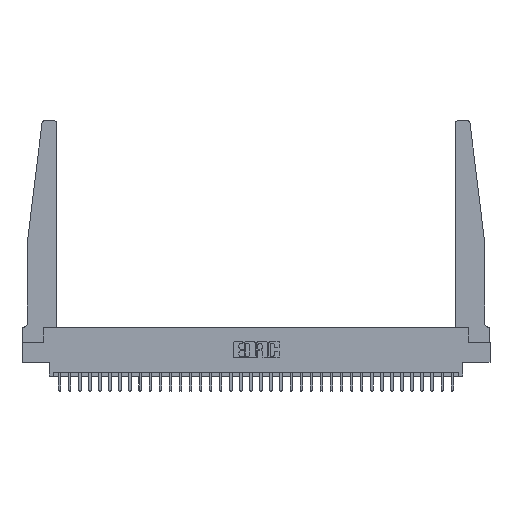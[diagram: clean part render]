
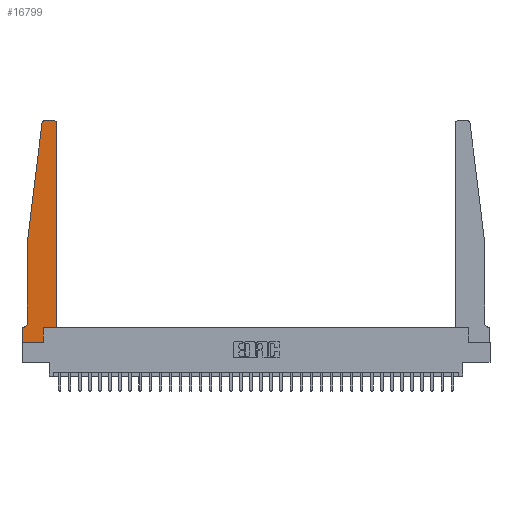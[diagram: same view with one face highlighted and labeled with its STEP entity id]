
A CAD part, top view. The second image highlights one B-rep face of the part: STEP entity #16799.
In plain terms, the highlighted planar face has unit normal (0, 0, 1).
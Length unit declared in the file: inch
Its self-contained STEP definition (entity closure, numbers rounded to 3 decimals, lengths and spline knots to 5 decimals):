
#183 = DIRECTION ( 'NONE',  ( 0., -1., 0. ) ) ;
#861 = EDGE_CURVE ( 'NONE', #28342, #23080, #4961, .T. ) ;
#1262 = VECTOR ( 'NONE', #183, 39.37008 ) ;
#2388 = VERTEX_POINT ( 'NONE', #28001 ) ;
#2410 = DIRECTION ( 'NONE',  ( -1., 0., 0. ) ) ;
#2727 = CARTESIAN_POINT ( 'NONE',  ( 0.2605, 0., 0.37 ) ) ;
#2827 = VECTOR ( 'NONE', #9152, 39.37008 ) ;
#3129 = VERTEX_POINT ( 'NONE', #16796 ) ;
#3364 = EDGE_CURVE ( 'NONE', #8021, #3392, #20960, .T. ) ;
#3392 = VERTEX_POINT ( 'NONE', #20138 ) ;
#3510 = DIRECTION ( 'NONE',  ( -0.122, -0.992, 0. ) ) ;
#4955 = CARTESIAN_POINT ( 'NONE',  ( 0.25, 2.75, 0.37 ) ) ;
#4961 = LINE ( 'NONE', #15987, #18856 ) ;
#5019 = VERTEX_POINT ( 'NONE', #28207 ) ;
#5576 = EDGE_CURVE ( 'NONE', #5019, #2388, #22667, .T. ) ;
#5673 = EDGE_CURVE ( 'NONE', #22853, #3129, #7489, .T. ) ;
#5853 = CARTESIAN_POINT ( 'NONE',  ( 0.065, 1.25, 0.37 ) ) ;
#6017 = ORIENTED_EDGE ( 'NONE', *, *, #10402, .T. ) ;
#6087 = CARTESIAN_POINT ( 'NONE',  ( 0.395, 2.72, 0.37 ) ) ;
#7252 = ORIENTED_EDGE ( 'NONE', *, *, #5576, .T. ) ;
#7489 = LINE ( 'NONE', #21246, #20468 ) ;
#7594 = ORIENTED_EDGE ( 'NONE', *, *, #5673, .T. ) ;
#7790 = VECTOR ( 'NONE', #22887, 39.37008 ) ;
#8021 = VERTEX_POINT ( 'NONE', #10655 ) ;
#8099 = CARTESIAN_POINT ( 'NONE',  ( 0.27653, 2.72, 0.37 ) ) ;
#8531 = LINE ( 'NONE', #4955, #20725 ) ;
#8535 = CARTESIAN_POINT ( 'NONE',  ( 0.015, 0.2375, 0.37 ) ) ;
#8607 = DIRECTION ( 'NONE',  ( 1., 0., 0. ) ) ;
#8812 = PLANE ( 'NONE',  #18573 ) ;
#9152 = DIRECTION ( 'NONE',  ( -1., 0., 0. ) ) ;
#9155 = DIRECTION ( 'NONE',  ( 1., 0., 0. ) ) ;
#9532 = LINE ( 'NONE', #18881, #2827 ) ;
#10249 = CARTESIAN_POINT ( 'NONE',  ( 0., 0., 0.37 ) ) ;
#10363 = LINE ( 'NONE', #22109, #22428 ) ;
#10402 = EDGE_CURVE ( 'NONE', #22274, #21176, #17820, .T. ) ;
#10571 = VERTEX_POINT ( 'NONE', #30438 ) ;
#10602 = DIRECTION ( 'NONE',  ( 1., 0., 0. ) ) ;
#10638 = ORIENTED_EDGE ( 'NONE', *, *, #13900, .T. ) ;
#10655 = CARTESIAN_POINT ( 'NONE',  ( 0., 0.1875, 0.37 ) ) ;
#11037 = DIRECTION ( 'NONE',  ( -1., 0., 0. ) ) ;
#11327 = DIRECTION ( 'NONE',  ( 1., 0., 0. ) ) ;
#12729 = ORIENTED_EDGE ( 'NONE', *, *, #31238, .T. ) ;
#13421 = CARTESIAN_POINT ( 'NONE',  ( 0.425, 0.18, 0.37 ) ) ;
#13825 = CARTESIAN_POINT ( 'NONE',  ( 0.24675, 2.72367, 0.37 ) ) ;
#13900 = EDGE_CURVE ( 'NONE', #24405, #22853, #19134, .T. ) ;
#14165 = CARTESIAN_POINT ( 'NONE',  ( 0.2605, 0.18, 0.37 ) ) ;
#14220 = CARTESIAN_POINT ( 'NONE',  ( 0.065, 0.2375, 0.37 ) ) ;
#15987 = CARTESIAN_POINT ( 'NONE',  ( 0.065, 1.25, 0.37 ) ) ;
#16172 = CARTESIAN_POINT ( 'NONE',  ( 0., 0.1875, 0.37 ) ) ;
#16620 = DIRECTION ( 'NONE',  ( 0., 1., 0. ) ) ;
#16796 = CARTESIAN_POINT ( 'NONE',  ( 0.425, 0.18, 0.37 ) ) ;
#16799 = ADVANCED_FACE ( 'NONE', ( #20172 ), #8812, .T. ) ;
#17820 = CIRCLE ( 'NONE', #19239, 0.05 ) ;
#17997 = EDGE_CURVE ( 'NONE', #3129, #5019, #25944, .T. ) ;
#18573 = AXIS2_PLACEMENT_3D ( 'NONE', #16172, #25641, #11327 ) ;
#18640 = CARTESIAN_POINT ( 'NONE',  ( 0.2605, 0.18, 0.37 ) ) ;
#18856 = VECTOR ( 'NONE', #3510, 39.37008 ) ;
#18881 = CARTESIAN_POINT ( 'NONE',  ( 0.065, 0.1875, 0.37 ) ) ;
#19134 = LINE ( 'NONE', #14165, #30805 ) ;
#19157 = EDGE_CURVE ( 'NONE', #23080, #22274, #20033, .T. ) ;
#19239 = AXIS2_PLACEMENT_3D ( 'NONE', #8535, #25369, #11037 ) ;
#19448 = CARTESIAN_POINT ( 'NONE',  ( 0.065, 1.25, 0.37 ) ) ;
#20033 = LINE ( 'NONE', #5853, #7790 ) ;
#20138 = CARTESIAN_POINT ( 'NONE',  ( 0., 0., 0.37 ) ) ;
#20162 = ORIENTED_EDGE ( 'NONE', *, *, #28421, .T. ) ;
#20172 = FACE_OUTER_BOUND ( 'NONE', #23894, .T. ) ;
#20468 = VECTOR ( 'NONE', #9155, 39.37008 ) ;
#20725 = VECTOR ( 'NONE', #2410, 39.37008 ) ;
#20960 = LINE ( 'NONE', #10249, #1262 ) ;
#21065 = CIRCLE ( 'NONE', #27899, 0.03 ) ;
#21176 = VERTEX_POINT ( 'NONE', #21449 ) ;
#21246 = CARTESIAN_POINT ( 'NONE',  ( 0.425, 0.18, 0.37 ) ) ;
#21449 = CARTESIAN_POINT ( 'NONE',  ( 0.015, 0.1875, 0.37 ) ) ;
#22109 = CARTESIAN_POINT ( 'NONE',  ( 0., 0., 0.37 ) ) ;
#22274 = VERTEX_POINT ( 'NONE', #14220 ) ;
#22428 = VECTOR ( 'NONE', #24458, 39.37008 ) ;
#22667 = CIRCLE ( 'NONE', #26826, 0.03 ) ;
#22853 = VERTEX_POINT ( 'NONE', #18640 ) ;
#22887 = DIRECTION ( 'NONE',  ( 0., -1., 0. ) ) ;
#23080 = VERTEX_POINT ( 'NONE', #19448 ) ;
#23092 = DIRECTION ( 'NONE',  ( 0., 0., 1. ) ) ;
#23115 = ORIENTED_EDGE ( 'NONE', *, *, #27956, .T. ) ;
#23894 = EDGE_LOOP ( 'NONE', ( #12729, #26189, #24034, #30651, #6017, #20162, #25871, #23115, #10638, #7594, #28337, #7252 ) ) ;
#24034 = ORIENTED_EDGE ( 'NONE', *, *, #861, .T. ) ;
#24405 = VERTEX_POINT ( 'NONE', #2727 ) ;
#24458 = DIRECTION ( 'NONE',  ( 1., 0., 0. ) ) ;
#24955 = DIRECTION ( 'NONE',  ( 0., 0., 1. ) ) ;
#25369 = DIRECTION ( 'NONE',  ( 0., 0., -1. ) ) ;
#25641 = DIRECTION ( 'NONE',  ( 0., 0., 1. ) ) ;
#25871 = ORIENTED_EDGE ( 'NONE', *, *, #3364, .T. ) ;
#25944 = LINE ( 'NONE', #13421, #26676 ) ;
#26189 = ORIENTED_EDGE ( 'NONE', *, *, #26221, .T. ) ;
#26221 = EDGE_CURVE ( 'NONE', #10571, #28342, #21065, .T. ) ;
#26676 = VECTOR ( 'NONE', #29946, 39.37008 ) ;
#26826 = AXIS2_PLACEMENT_3D ( 'NONE', #6087, #23092, #8607 ) ;
#27899 = AXIS2_PLACEMENT_3D ( 'NONE', #8099, #24955, #10602 ) ;
#27956 = EDGE_CURVE ( 'NONE', #3392, #24405, #10363, .T. ) ;
#28001 = CARTESIAN_POINT ( 'NONE',  ( 0.395, 2.75, 0.37 ) ) ;
#28207 = CARTESIAN_POINT ( 'NONE',  ( 0.425, 2.72, 0.37 ) ) ;
#28337 = ORIENTED_EDGE ( 'NONE', *, *, #17997, .T. ) ;
#28342 = VERTEX_POINT ( 'NONE', #13825 ) ;
#28421 = EDGE_CURVE ( 'NONE', #21176, #8021, #9532, .T. ) ;
#29946 = DIRECTION ( 'NONE',  ( 0., 1., 0. ) ) ;
#30438 = CARTESIAN_POINT ( 'NONE',  ( 0.27653, 2.75, 0.37 ) ) ;
#30651 = ORIENTED_EDGE ( 'NONE', *, *, #19157, .T. ) ;
#30805 = VECTOR ( 'NONE', #16620, 39.37008 ) ;
#31238 = EDGE_CURVE ( 'NONE', #2388, #10571, #8531, .T. ) ;
